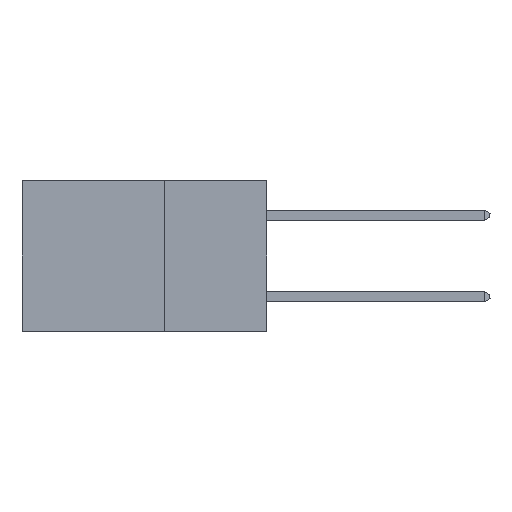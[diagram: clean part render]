
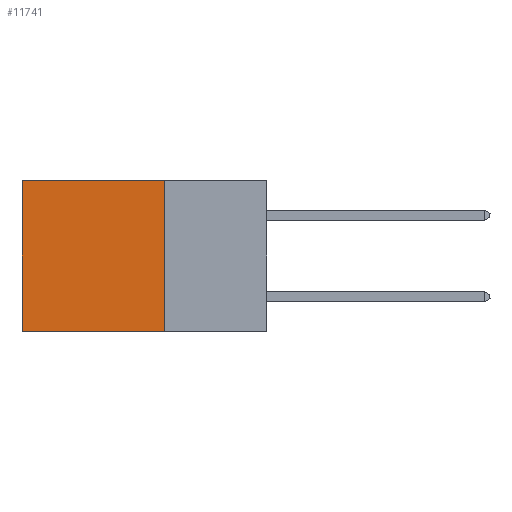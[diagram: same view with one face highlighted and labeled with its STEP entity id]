
A CAD part, left-side view. The second image highlights one B-rep face of the part: STEP entity #11741.
In plain terms, the highlighted planar face has unit normal (-1, 0, 0).
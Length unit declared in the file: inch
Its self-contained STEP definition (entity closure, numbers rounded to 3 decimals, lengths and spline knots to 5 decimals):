
#641 = AXIS2_PLACEMENT_3D ( 'NONE', #2485, #39479, #30418 ) ;
#2485 = CARTESIAN_POINT ( 'NONE',  ( 0.2875, 0.25, 0. ) ) ;
#3728 = ORIENTED_EDGE ( 'NONE', *, *, #30207, .F. ) ;
#4849 = CARTESIAN_POINT ( 'NONE',  ( 0.2875, 0.25, 0. ) ) ;
#6092 = EDGE_CURVE ( 'NONE', #20418, #37958, #39883, .T. ) ;
#7174 = LINE ( 'NONE', #35506, #14545 ) ;
#11377 = EDGE_CURVE ( 'NONE', #38358, #17443, #19727, .T. ) ;
#11741 = ADVANCED_FACE ( 'NONE', ( #37915 ), #27331, .F. ) ;
#14236 = LINE ( 'NONE', #27602, #20531 ) ;
#14545 = VECTOR ( 'NONE', #20186, 39.37008 ) ;
#15308 = DIRECTION ( 'NONE',  ( 0., 1., 0. ) ) ;
#16370 = VECTOR ( 'NONE', #26586, 39.37008 ) ;
#16437 = CARTESIAN_POINT ( 'NONE',  ( 0.2875, 0.6, 0. ) ) ;
#17030 = ORIENTED_EDGE ( 'NONE', *, *, #6092, .F. ) ;
#17443 = VERTEX_POINT ( 'NONE', #27839 ) ;
#18229 = CARTESIAN_POINT ( 'NONE',  ( 0.2875, 0.25, -0.37 ) ) ;
#19154 = EDGE_CURVE ( 'NONE', #20418, #38358, #7174, .T. ) ;
#19565 = DIRECTION ( 'NONE',  ( 0., 0., -1. ) ) ;
#19727 = LINE ( 'NONE', #16437, #35113 ) ;
#20186 = DIRECTION ( 'NONE',  ( 0., 1., 0. ) ) ;
#20418 = VERTEX_POINT ( 'NONE', #27241 ) ;
#20531 = VECTOR ( 'NONE', #15308, 39.37008 ) ;
#20746 = ORIENTED_EDGE ( 'NONE', *, *, #11377, .T. ) ;
#24984 = ORIENTED_EDGE ( 'NONE', *, *, #19154, .T. ) ;
#26586 = DIRECTION ( 'NONE',  ( 0., 0., -1. ) ) ;
#27241 = CARTESIAN_POINT ( 'NONE',  ( 0.2875, 0.25, 0. ) ) ;
#27331 = PLANE ( 'NONE',  #641 ) ;
#27602 = CARTESIAN_POINT ( 'NONE',  ( 0.2875, 0.25, -0.37 ) ) ;
#27781 = CARTESIAN_POINT ( 'NONE',  ( 0.2875, 0.6, 0. ) ) ;
#27839 = CARTESIAN_POINT ( 'NONE',  ( 0.2875, 0.6, -0.37 ) ) ;
#30207 = EDGE_CURVE ( 'NONE', #37958, #17443, #14236, .T. ) ;
#30418 = DIRECTION ( 'NONE',  ( 0., 0., -1. ) ) ;
#32381 = EDGE_LOOP ( 'NONE', ( #20746, #3728, #17030, #24984 ) ) ;
#35113 = VECTOR ( 'NONE', #19565, 39.37008 ) ;
#35506 = CARTESIAN_POINT ( 'NONE',  ( 0.2875, 0.25, 0. ) ) ;
#37915 = FACE_OUTER_BOUND ( 'NONE', #32381, .T. ) ;
#37958 = VERTEX_POINT ( 'NONE', #18229 ) ;
#38358 = VERTEX_POINT ( 'NONE', #27781 ) ;
#39479 = DIRECTION ( 'NONE',  ( 1., 0., 0. ) ) ;
#39883 = LINE ( 'NONE', #4849, #16370 ) ;
